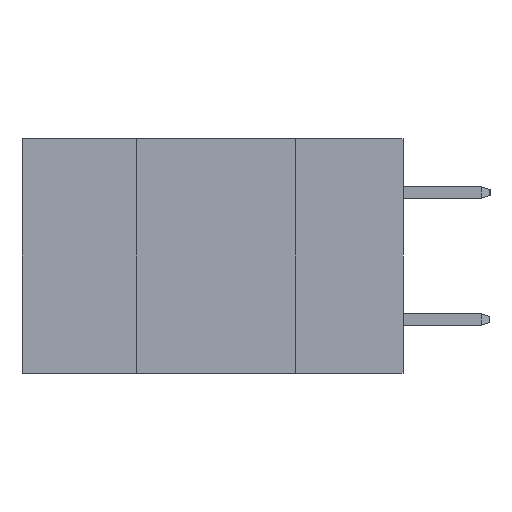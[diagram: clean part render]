
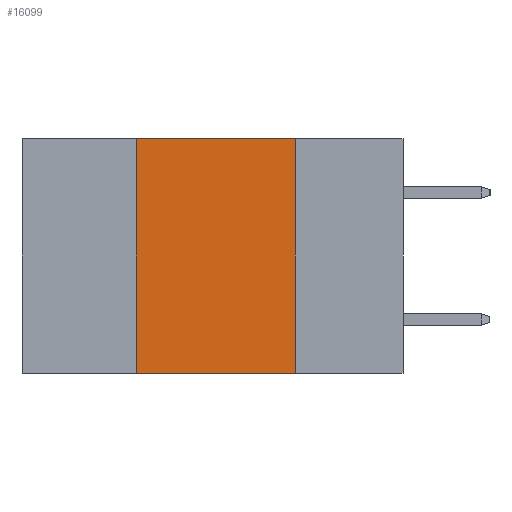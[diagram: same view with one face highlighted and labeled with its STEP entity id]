
A CAD part, left-side view. The second image highlights one B-rep face of the part: STEP entity #16099.
In plain terms, the highlighted planar face has unit normal (-1, 0, 0).
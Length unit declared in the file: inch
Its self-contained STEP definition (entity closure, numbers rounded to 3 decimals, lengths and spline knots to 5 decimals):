
#1058 = VECTOR ( 'NONE', #42491, 39.37008 ) ;
#3148 = VERTEX_POINT ( 'NONE', #47364 ) ;
#4778 = DIRECTION ( 'NONE',  ( 0., 0., -1. ) ) ;
#4819 = VECTOR ( 'NONE', #4778, 39.37008 ) ;
#6640 = AXIS2_PLACEMENT_3D ( 'NONE', #18127, #36132, #21009 ) ;
#6839 = VERTEX_POINT ( 'NONE', #19124 ) ;
#8725 = CARTESIAN_POINT ( 'NONE',  ( 0., 0.6, 0. ) ) ;
#8856 = LINE ( 'NONE', #38355, #4819 ) ;
#9755 = EDGE_CURVE ( 'NONE', #3148, #38262, #8856, .T. ) ;
#10169 = CARTESIAN_POINT ( 'NONE',  ( 0., 0.17, -0.37 ) ) ;
#14764 = PLANE ( 'NONE',  #6640 ) ;
#14847 = ORIENTED_EDGE ( 'NONE', *, *, #40197, .F. ) ;
#16099 = ADVANCED_FACE ( 'NONE', ( #39740 ), #14764, .F. ) ;
#18127 = CARTESIAN_POINT ( 'NONE',  ( 0., 0.6, 0. ) ) ;
#18309 = EDGE_CURVE ( 'NONE', #6839, #3148, #45423, .T. ) ;
#18971 = CARTESIAN_POINT ( 'NONE',  ( 0., 0.42, -0.37 ) ) ;
#19124 = CARTESIAN_POINT ( 'NONE',  ( 0., 0.42, 0. ) ) ;
#21009 = DIRECTION ( 'NONE',  ( 0., 0., -1. ) ) ;
#22119 = VERTEX_POINT ( 'NONE', #18971 ) ;
#24979 = LINE ( 'NONE', #39621, #1058 ) ;
#25705 = LINE ( 'NONE', #37222, #27277 ) ;
#26164 = DIRECTION ( 'NONE',  ( 0., 0., 1. ) ) ;
#27277 = VECTOR ( 'NONE', #26164, 39.37008 ) ;
#32866 = VECTOR ( 'NONE', #38005, 39.37008 ) ;
#33277 = ORIENTED_EDGE ( 'NONE', *, *, #18309, .F. ) ;
#33901 = ORIENTED_EDGE ( 'NONE', *, *, #35436, .T. ) ;
#35436 = EDGE_CURVE ( 'NONE', #22119, #38262, #24979, .T. ) ;
#36132 = DIRECTION ( 'NONE',  ( 1., 0., 0. ) ) ;
#37222 = CARTESIAN_POINT ( 'NONE',  ( 0., 0.42, 0. ) ) ;
#38005 = DIRECTION ( 'NONE',  ( 0., -1., 0. ) ) ;
#38094 = ORIENTED_EDGE ( 'NONE', *, *, #9755, .F. ) ;
#38262 = VERTEX_POINT ( 'NONE', #10169 ) ;
#38355 = CARTESIAN_POINT ( 'NONE',  ( 0., 0.17, 0. ) ) ;
#39621 = CARTESIAN_POINT ( 'NONE',  ( 0., 0.6, -0.37 ) ) ;
#39740 = FACE_OUTER_BOUND ( 'NONE', #39854, .T. ) ;
#39854 = EDGE_LOOP ( 'NONE', ( #38094, #33277, #14847, #33901 ) ) ;
#40197 = EDGE_CURVE ( 'NONE', #22119, #6839, #25705, .T. ) ;
#42491 = DIRECTION ( 'NONE',  ( 0., -1., 0. ) ) ;
#45423 = LINE ( 'NONE', #8725, #32866 ) ;
#47364 = CARTESIAN_POINT ( 'NONE',  ( 0., 0.17, 0. ) ) ;
